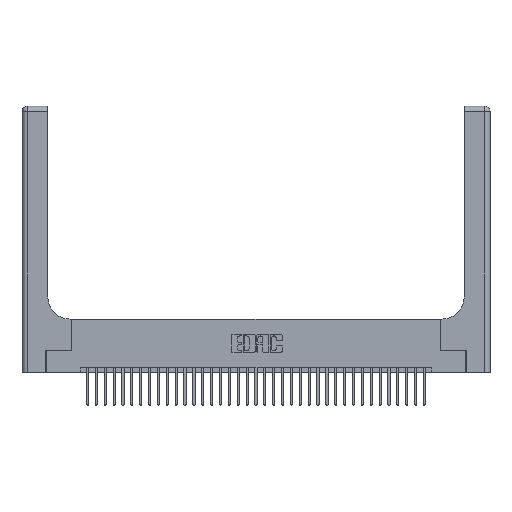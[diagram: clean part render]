
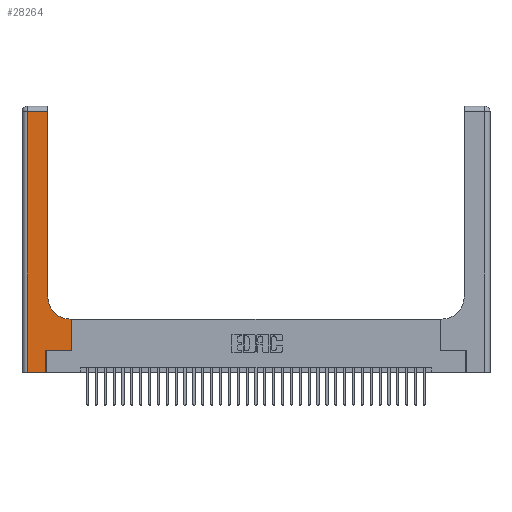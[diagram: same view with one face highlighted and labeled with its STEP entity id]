
A CAD part, top view. The second image highlights one B-rep face of the part: STEP entity #28264.
In plain terms, the highlighted planar face has unit normal (0, 0, 1).
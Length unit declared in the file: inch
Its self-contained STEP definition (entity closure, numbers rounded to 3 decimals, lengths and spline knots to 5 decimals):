
#177 = LINE ( 'NONE', #10390, #31588 ) ;
#350 = EDGE_CURVE ( 'NONE', #12896, #24730, #7062, .T. ) ;
#684 = DIRECTION ( 'NONE',  ( 1., 0., 0. ) ) ;
#964 = CARTESIAN_POINT ( 'NONE',  ( 0.2915, 0.85, 0.37 ) ) ;
#1201 = FACE_OUTER_BOUND ( 'NONE', #32858, .T. ) ;
#1397 = CARTESIAN_POINT ( 'NONE',  ( 0.06, 0., 0.37 ) ) ;
#1778 = EDGE_CURVE ( 'NONE', #24737, #11269, #12055, .T. ) ;
#2041 = VERTEX_POINT ( 'NONE', #2523 ) ;
#2370 = EDGE_CURVE ( 'NONE', #24730, #2041, #26870, .T. ) ;
#2523 = CARTESIAN_POINT ( 'NONE',  ( 0.5585, 0.6, 0.37 ) ) ;
#2669 = EDGE_CURVE ( 'NONE', #11269, #28948, #25604, .T. ) ;
#4658 = VECTOR ( 'NONE', #16558, 39.37008 ) ;
#6841 = CARTESIAN_POINT ( 'NONE',  ( 0.5585, 0.25, 0.37 ) ) ;
#6937 = CARTESIAN_POINT ( 'NONE',  ( 0.2915, 3., 0.37 ) ) ;
#7062 = LINE ( 'NONE', #30426, #31837 ) ;
#7579 = AXIS2_PLACEMENT_3D ( 'NONE', #30879, #22588, #17683 ) ;
#8878 = CARTESIAN_POINT ( 'NONE',  ( 0.06, 2.94, 0.37 ) ) ;
#9234 = CARTESIAN_POINT ( 'NONE',  ( 0.269, 0.25, 0.37 ) ) ;
#9353 = CARTESIAN_POINT ( 'NONE',  ( 0.269, 0., 0.37 ) ) ;
#9425 = AXIS2_PLACEMENT_3D ( 'NONE', #20807, #12141, #31688 ) ;
#9595 = LINE ( 'NONE', #9353, #22737 ) ;
#10390 = CARTESIAN_POINT ( 'NONE',  ( 0.2915, 0.6, 0.37 ) ) ;
#11269 = VERTEX_POINT ( 'NONE', #1397 ) ;
#12055 = LINE ( 'NONE', #21318, #4658 ) ;
#12141 = DIRECTION ( 'NONE',  ( 0., 0., -1. ) ) ;
#12343 = DIRECTION ( 'NONE',  ( 0., 1., 0. ) ) ;
#12499 = VECTOR ( 'NONE', #18748, 39.37008 ) ;
#12575 = CARTESIAN_POINT ( 'NONE',  ( 0.5415, 0.6, 0.37 ) ) ;
#12896 = VERTEX_POINT ( 'NONE', #9234 ) ;
#13036 = ORIENTED_EDGE ( 'NONE', *, *, #2669, .T. ) ;
#13204 = ORIENTED_EDGE ( 'NONE', *, *, #26530, .T. ) ;
#13430 = EDGE_CURVE ( 'NONE', #28816, #19373, #19378, .T. ) ;
#14079 = ORIENTED_EDGE ( 'NONE', *, *, #13430, .T. ) ;
#15175 = ORIENTED_EDGE ( 'NONE', *, *, #29012, .T. ) ;
#15297 = VECTOR ( 'NONE', #15492, 39.37008 ) ;
#15492 = DIRECTION ( 'NONE',  ( 0., 1., 0. ) ) ;
#16040 = CARTESIAN_POINT ( 'NONE',  ( 0., 0., 0.37 ) ) ;
#16101 = DIRECTION ( 'NONE',  ( -1., 0., 0. ) ) ;
#16558 = DIRECTION ( 'NONE',  ( 0., -1., 0. ) ) ;
#16945 = VERTEX_POINT ( 'NONE', #31531 ) ;
#17071 = LINE ( 'NONE', #6937, #15297 ) ;
#17683 = DIRECTION ( 'NONE',  ( 1., 0., 0. ) ) ;
#18720 = ORIENTED_EDGE ( 'NONE', *, *, #350, .T. ) ;
#18727 = DIRECTION ( 'NONE',  ( -1., 0., 0. ) ) ;
#18748 = DIRECTION ( 'NONE',  ( 1., 0., 0. ) ) ;
#19373 = VERTEX_POINT ( 'NONE', #964 ) ;
#19378 = CIRCLE ( 'NONE', #7579, 0.25 ) ;
#20654 = ORIENTED_EDGE ( 'NONE', *, *, #2370, .T. ) ;
#20807 = CARTESIAN_POINT ( 'NONE',  ( 0., 3., 0.37 ) ) ;
#20998 = DIRECTION ( 'NONE',  ( 0., 1., 0. ) ) ;
#21318 = CARTESIAN_POINT ( 'NONE',  ( 0.06, 3., 0.37 ) ) ;
#22588 = DIRECTION ( 'NONE',  ( 0., 0., -1. ) ) ;
#22737 = VECTOR ( 'NONE', #20998, 39.37008 ) ;
#24158 = LINE ( 'NONE', #30139, #35551 ) ;
#24730 = VERTEX_POINT ( 'NONE', #30891 ) ;
#24737 = VERTEX_POINT ( 'NONE', #8878 ) ;
#24996 = ORIENTED_EDGE ( 'NONE', *, *, #26548, .T. ) ;
#25562 = EDGE_CURVE ( 'NONE', #16945, #24737, #24158, .T. ) ;
#25604 = LINE ( 'NONE', #16040, #12499 ) ;
#26530 = EDGE_CURVE ( 'NONE', #28948, #12896, #9595, .T. ) ;
#26548 = EDGE_CURVE ( 'NONE', #19373, #16945, #17071, .T. ) ;
#26870 = LINE ( 'NONE', #6841, #30403 ) ;
#28264 = ADVANCED_FACE ( 'NONE', ( #1201 ), #28856, .F. ) ;
#28816 = VERTEX_POINT ( 'NONE', #12575 ) ;
#28856 = PLANE ( 'NONE',  #9425 ) ;
#28867 = ORIENTED_EDGE ( 'NONE', *, *, #1778, .T. ) ;
#28948 = VERTEX_POINT ( 'NONE', #35597 ) ;
#29012 = EDGE_CURVE ( 'NONE', #2041, #28816, #177, .T. ) ;
#30139 = CARTESIAN_POINT ( 'NONE',  ( 0., 2.94, 0.37 ) ) ;
#30403 = VECTOR ( 'NONE', #12343, 39.37008 ) ;
#30426 = CARTESIAN_POINT ( 'NONE',  ( 0.269, 0.25, 0.37 ) ) ;
#30879 = CARTESIAN_POINT ( 'NONE',  ( 0.5415, 0.85, 0.37 ) ) ;
#30891 = CARTESIAN_POINT ( 'NONE',  ( 0.5585, 0.25, 0.37 ) ) ;
#31531 = CARTESIAN_POINT ( 'NONE',  ( 0.2915, 2.94, 0.37 ) ) ;
#31588 = VECTOR ( 'NONE', #18727, 39.37008 ) ;
#31688 = DIRECTION ( 'NONE',  ( -1., 0., 0. ) ) ;
#31837 = VECTOR ( 'NONE', #684, 39.37008 ) ;
#32858 = EDGE_LOOP ( 'NONE', ( #24996, #34018, #28867, #13036, #13204, #18720, #20654, #15175, #14079 ) ) ;
#34018 = ORIENTED_EDGE ( 'NONE', *, *, #25562, .T. ) ;
#35551 = VECTOR ( 'NONE', #16101, 39.37008 ) ;
#35597 = CARTESIAN_POINT ( 'NONE',  ( 0.269, 0., 0.37 ) ) ;
